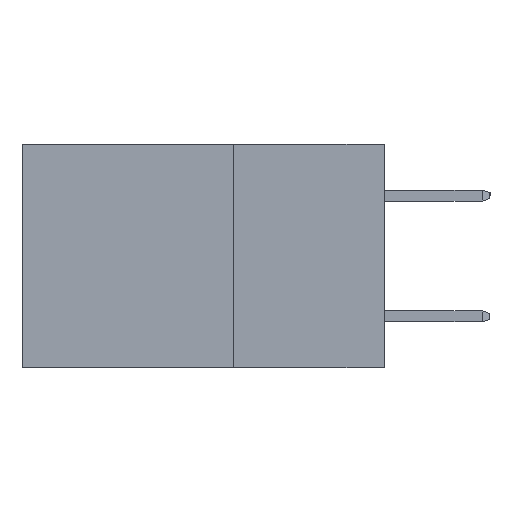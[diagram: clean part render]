
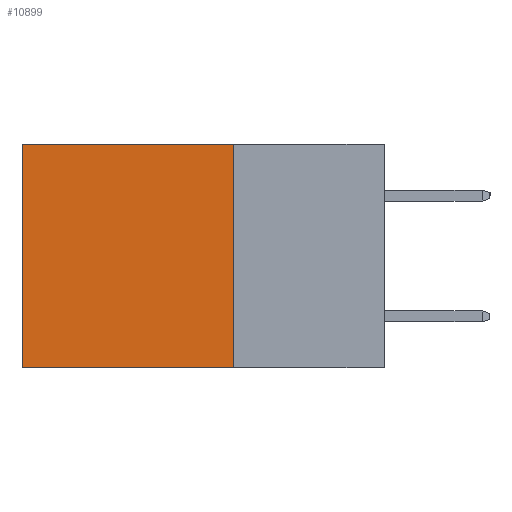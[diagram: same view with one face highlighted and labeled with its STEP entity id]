
A CAD part, left-side view. The second image highlights one B-rep face of the part: STEP entity #10899.
In plain terms, the highlighted planar face has unit normal (-1, 0, 0).
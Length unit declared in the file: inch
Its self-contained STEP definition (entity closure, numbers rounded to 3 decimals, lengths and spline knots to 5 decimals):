
#74 = EDGE_CURVE ( 'NONE', #1187, #7781, #10710, .T. ) ;
#99 = VERTEX_POINT ( 'NONE', #3272 ) ;
#447 = ORIENTED_EDGE ( 'NONE', *, *, #2342, .T. ) ;
#1161 = FACE_OUTER_BOUND ( 'NONE', #6649, .T. ) ;
#1187 = VERTEX_POINT ( 'NONE', #8343 ) ;
#1224 = DIRECTION ( 'NONE',  ( 0., 0., -1. ) ) ;
#1291 = DIRECTION ( 'NONE',  ( 0., 1., 0. ) ) ;
#1438 = DIRECTION ( 'NONE',  ( 0., 1., 0. ) ) ;
#1741 = VERTEX_POINT ( 'NONE', #8735 ) ;
#2002 = ORIENTED_EDGE ( 'NONE', *, *, #12673, .F. ) ;
#2342 = EDGE_CURVE ( 'NONE', #99, #1741, #11377, .T. ) ;
#3144 = AXIS2_PLACEMENT_3D ( 'NONE', #6363, #12560, #1224 ) ;
#3272 = CARTESIAN_POINT ( 'NONE',  ( 0.2615, 0.25, 0. ) ) ;
#3541 = CARTESIAN_POINT ( 'NONE',  ( 0.2615, 0.25, -0.37 ) ) ;
#3732 = ORIENTED_EDGE ( 'NONE', *, *, #5846, .T. ) ;
#3971 = VECTOR ( 'NONE', #12557, 39.37008 ) ;
#4261 = LINE ( 'NONE', #10494, #3971 ) ;
#4391 = LINE ( 'NONE', #7499, #13157 ) ;
#5846 = EDGE_CURVE ( 'NONE', #1741, #7781, #4261, .T. ) ;
#6363 = CARTESIAN_POINT ( 'NONE',  ( 0.2615, 0.25, -0.37 ) ) ;
#6649 = EDGE_LOOP ( 'NONE', ( #3732, #9739, #2002, #447 ) ) ;
#7129 = VECTOR ( 'NONE', #1291, 39.37008 ) ;
#7499 = CARTESIAN_POINT ( 'NONE',  ( 0.2615, 0.25, -0.37 ) ) ;
#7781 = VERTEX_POINT ( 'NONE', #12267 ) ;
#8343 = CARTESIAN_POINT ( 'NONE',  ( 0.2615, 0.25, -0.37 ) ) ;
#8403 = PLANE ( 'NONE',  #3144 ) ;
#8735 = CARTESIAN_POINT ( 'NONE',  ( 0.2615, 0.6, 0. ) ) ;
#8825 = VECTOR ( 'NONE', #1438, 39.37008 ) ;
#9351 = CARTESIAN_POINT ( 'NONE',  ( 0.2615, 0.25, 0. ) ) ;
#9739 = ORIENTED_EDGE ( 'NONE', *, *, #74, .F. ) ;
#10494 = CARTESIAN_POINT ( 'NONE',  ( 0.2615, 0.6, -0.37 ) ) ;
#10629 = DIRECTION ( 'NONE',  ( 0., 0., -1. ) ) ;
#10710 = LINE ( 'NONE', #3541, #8825 ) ;
#10899 = ADVANCED_FACE ( 'NONE', ( #1161 ), #8403, .F. ) ;
#11377 = LINE ( 'NONE', #9351, #7129 ) ;
#12267 = CARTESIAN_POINT ( 'NONE',  ( 0.2615, 0.6, -0.37 ) ) ;
#12557 = DIRECTION ( 'NONE',  ( 0., 0., -1. ) ) ;
#12560 = DIRECTION ( 'NONE',  ( 1., 0., 0. ) ) ;
#12673 = EDGE_CURVE ( 'NONE', #99, #1187, #4391, .T. ) ;
#13157 = VECTOR ( 'NONE', #10629, 39.37008 ) ;
